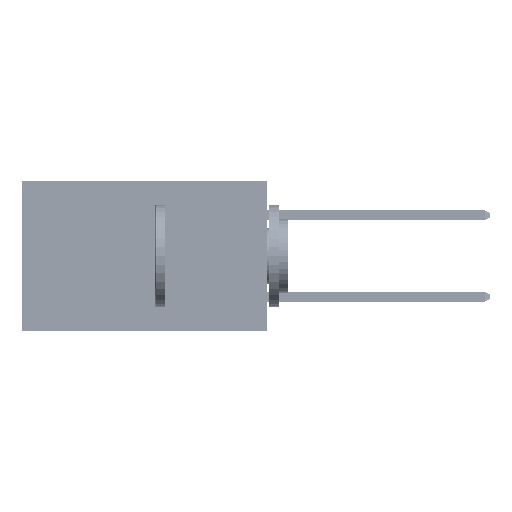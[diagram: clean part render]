
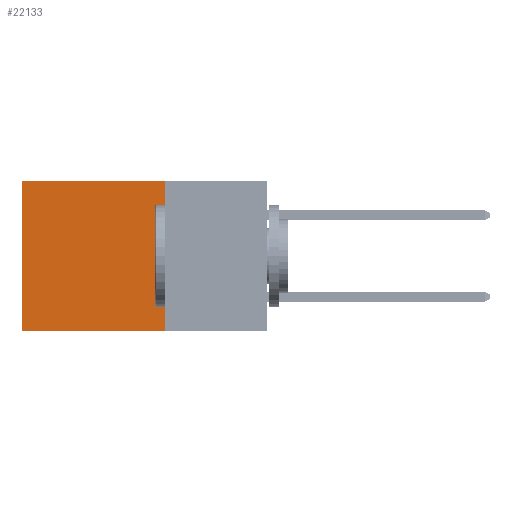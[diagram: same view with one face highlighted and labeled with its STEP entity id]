
A CAD part, left-side view. The second image highlights one B-rep face of the part: STEP entity #22133.
In plain terms, the highlighted planar face has unit normal (-1, 0, 0).
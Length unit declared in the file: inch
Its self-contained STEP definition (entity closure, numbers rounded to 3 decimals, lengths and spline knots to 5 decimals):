
#160 = EDGE_CURVE ( 'NONE', #12961, #22096, #6597, .T. ) ;
#2897 = VECTOR ( 'NONE', #10874, 39.37008 ) ;
#5036 = EDGE_CURVE ( 'NONE', #41054, #41960, #28456, .T. ) ;
#5304 = DIRECTION ( 'NONE',  ( 0., 0., -1. ) ) ;
#5398 = EDGE_CURVE ( 'NONE', #41960, #22096, #42302, .T. ) ;
#6597 = LINE ( 'NONE', #34299, #2897 ) ;
#8292 = ORIENTED_EDGE ( 'NONE', *, *, #12164, .F. ) ;
#8618 = CARTESIAN_POINT ( 'NONE',  ( 0.2875, 0.25, 0. ) ) ;
#9288 = CARTESIAN_POINT ( 'NONE',  ( 0.2875, 0.25, 0. ) ) ;
#10874 = DIRECTION ( 'NONE',  ( 0., 1., 0. ) ) ;
#12164 = EDGE_CURVE ( 'NONE', #41054, #12961, #37713, .T. ) ;
#12419 = CARTESIAN_POINT ( 'NONE',  ( 0.2875, 0.25, 0. ) ) ;
#12501 = VECTOR ( 'NONE', #21911, 39.37008 ) ;
#12677 = DIRECTION ( 'NONE',  ( 0., 0., -1. ) ) ;
#12961 = VERTEX_POINT ( 'NONE', #18101 ) ;
#14686 = FACE_OUTER_BOUND ( 'NONE', #29647, .T. ) ;
#17082 = VECTOR ( 'NONE', #5304, 39.37008 ) ;
#17383 = ORIENTED_EDGE ( 'NONE', *, *, #5398, .T. ) ;
#18101 = CARTESIAN_POINT ( 'NONE',  ( 0.2875, 0.25, -0.37 ) ) ;
#21911 = DIRECTION ( 'NONE',  ( 0., 0., -1. ) ) ;
#22096 = VERTEX_POINT ( 'NONE', #47302 ) ;
#22133 = ADVANCED_FACE ( 'NONE', ( #14686 ), #32145, .F. ) ;
#23647 = DIRECTION ( 'NONE',  ( 0., 1., 0. ) ) ;
#25070 = AXIS2_PLACEMENT_3D ( 'NONE', #8618, #36027, #12677 ) ;
#28456 = LINE ( 'NONE', #42911, #47741 ) ;
#29647 = EDGE_LOOP ( 'NONE', ( #17383, #44758, #8292, #38251 ) ) ;
#32145 = PLANE ( 'NONE',  #25070 ) ;
#34299 = CARTESIAN_POINT ( 'NONE',  ( 0.2875, 0.25, -0.37 ) ) ;
#36027 = DIRECTION ( 'NONE',  ( 1., 0., 0. ) ) ;
#37713 = LINE ( 'NONE', #9288, #17082 ) ;
#38251 = ORIENTED_EDGE ( 'NONE', *, *, #5036, .T. ) ;
#41054 = VERTEX_POINT ( 'NONE', #12419 ) ;
#41960 = VERTEX_POINT ( 'NONE', #48300 ) ;
#42302 = LINE ( 'NONE', #45019, #12501 ) ;
#42911 = CARTESIAN_POINT ( 'NONE',  ( 0.2875, 0.25, 0. ) ) ;
#44758 = ORIENTED_EDGE ( 'NONE', *, *, #160, .F. ) ;
#45019 = CARTESIAN_POINT ( 'NONE',  ( 0.2875, 0.6, 0. ) ) ;
#47302 = CARTESIAN_POINT ( 'NONE',  ( 0.2875, 0.6, -0.37 ) ) ;
#47741 = VECTOR ( 'NONE', #23647, 39.37008 ) ;
#48300 = CARTESIAN_POINT ( 'NONE',  ( 0.2875, 0.6, 0. ) ) ;
